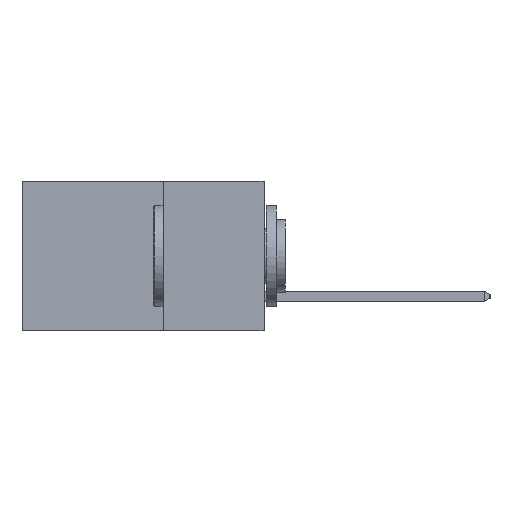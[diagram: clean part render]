
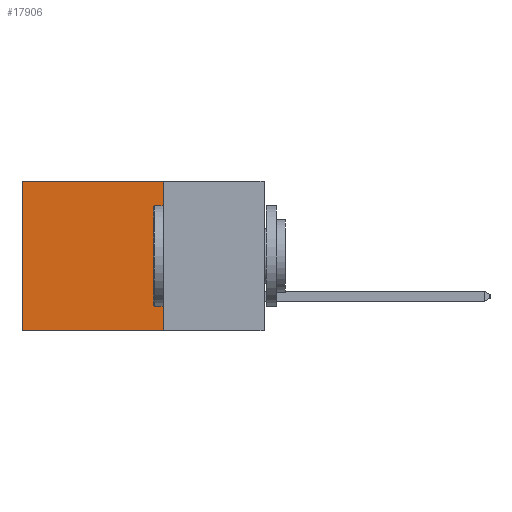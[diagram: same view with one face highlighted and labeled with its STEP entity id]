
A CAD part, left-side view. The second image highlights one B-rep face of the part: STEP entity #17906.
In plain terms, the highlighted planar face has unit normal (-1, 0, 0).
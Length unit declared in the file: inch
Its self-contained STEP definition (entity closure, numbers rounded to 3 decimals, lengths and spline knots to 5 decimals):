
#2058 = VERTEX_POINT ( 'NONE', #21667 ) ;
#2240 = ORIENTED_EDGE ( 'NONE', *, *, #13210, .T. ) ;
#2321 = LINE ( 'NONE', #9171, #17818 ) ;
#3419 = DIRECTION ( 'NONE',  ( 1., 0., 0. ) ) ;
#4284 = ORIENTED_EDGE ( 'NONE', *, *, #12724, .F. ) ;
#4503 = VECTOR ( 'NONE', #10962, 39.37008 ) ;
#4758 = VERTEX_POINT ( 'NONE', #16125 ) ;
#6506 = EDGE_CURVE ( 'NONE', #15850, #4758, #2321, .T. ) ;
#8508 = EDGE_LOOP ( 'NONE', ( #21624, #4284, #21792, #2240 ) ) ;
#9105 = DIRECTION ( 'NONE',  ( 0., 0., -1. ) ) ;
#9171 = CARTESIAN_POINT ( 'NONE',  ( 0.2615, 0.25, -0.37 ) ) ;
#9555 = CARTESIAN_POINT ( 'NONE',  ( 0.2615, 0.25, -0.37 ) ) ;
#9720 = VECTOR ( 'NONE', #16020, 39.37008 ) ;
#9962 = LINE ( 'NONE', #10796, #4503 ) ;
#10796 = CARTESIAN_POINT ( 'NONE',  ( 0.2615, 0.25, -0.37 ) ) ;
#10869 = CARTESIAN_POINT ( 'NONE',  ( 0.2615, 0.25, 0. ) ) ;
#10962 = DIRECTION ( 'NONE',  ( 0., 1., 0. ) ) ;
#11693 = EDGE_CURVE ( 'NONE', #20315, #2058, #24721, .T. ) ;
#12724 = EDGE_CURVE ( 'NONE', #4758, #2058, #9962, .T. ) ;
#13210 = EDGE_CURVE ( 'NONE', #15850, #20315, #14627, .T. ) ;
#14627 = LINE ( 'NONE', #23775, #19812 ) ;
#14910 = CARTESIAN_POINT ( 'NONE',  ( 0.2615, 0.6, -0.37 ) ) ;
#15544 = PLANE ( 'NONE',  #22547 ) ;
#15850 = VERTEX_POINT ( 'NONE', #10869 ) ;
#16020 = DIRECTION ( 'NONE',  ( 0., 0., -1. ) ) ;
#16125 = CARTESIAN_POINT ( 'NONE',  ( 0.2615, 0.25, -0.37 ) ) ;
#17498 = DIRECTION ( 'NONE',  ( 0., 0., -1. ) ) ;
#17818 = VECTOR ( 'NONE', #9105, 39.37008 ) ;
#17906 = ADVANCED_FACE ( 'NONE', ( #21203 ), #15544, .F. ) ;
#19812 = VECTOR ( 'NONE', #23727, 39.37008 ) ;
#20315 = VERTEX_POINT ( 'NONE', #20480 ) ;
#20480 = CARTESIAN_POINT ( 'NONE',  ( 0.2615, 0.6, 0. ) ) ;
#21203 = FACE_OUTER_BOUND ( 'NONE', #8508, .T. ) ;
#21624 = ORIENTED_EDGE ( 'NONE', *, *, #11693, .T. ) ;
#21667 = CARTESIAN_POINT ( 'NONE',  ( 0.2615, 0.6, -0.37 ) ) ;
#21792 = ORIENTED_EDGE ( 'NONE', *, *, #6506, .F. ) ;
#22547 = AXIS2_PLACEMENT_3D ( 'NONE', #9555, #3419, #17498 ) ;
#23727 = DIRECTION ( 'NONE',  ( 0., 1., 0. ) ) ;
#23775 = CARTESIAN_POINT ( 'NONE',  ( 0.2615, 0.25, 0. ) ) ;
#24721 = LINE ( 'NONE', #14910, #9720 ) ;
